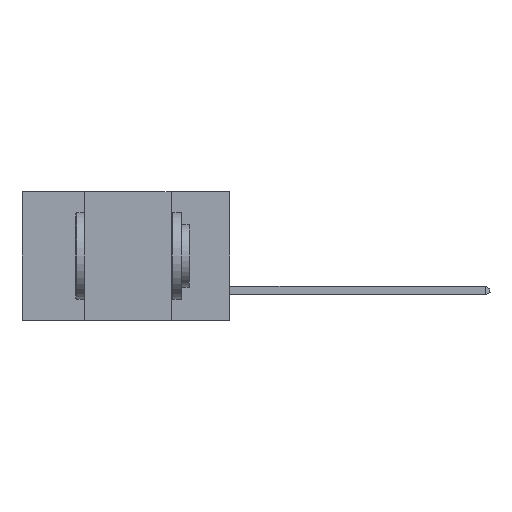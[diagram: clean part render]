
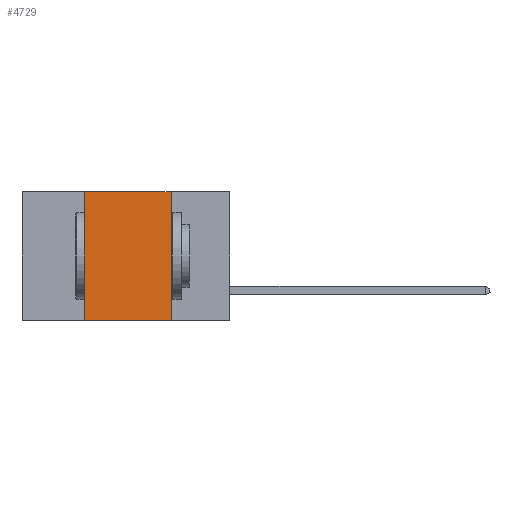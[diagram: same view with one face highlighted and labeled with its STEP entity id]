
A CAD part, left-side view. The second image highlights one B-rep face of the part: STEP entity #4729.
In plain terms, the highlighted planar face has unit normal (-1, 0, 0).
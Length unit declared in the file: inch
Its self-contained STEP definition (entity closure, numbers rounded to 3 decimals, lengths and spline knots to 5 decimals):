
#10 = ORIENTED_EDGE ( 'NONE', *, *, #11456, .F. ) ;
#204 = EDGE_CURVE ( 'NONE', #10013, #543, #9078, .T. ) ;
#543 = VERTEX_POINT ( 'NONE', #5342 ) ;
#908 = DIRECTION ( 'NONE',  ( 0., -1., 0. ) ) ;
#931 = DIRECTION ( 'NONE',  ( 0., 0., -1. ) ) ;
#1686 = DIRECTION ( 'NONE',  ( 0., 0., 1. ) ) ;
#1840 = CARTESIAN_POINT ( 'NONE',  ( 0., 0.42, -0.37 ) ) ;
#2018 = DIRECTION ( 'NONE',  ( 0., 0., -1. ) ) ;
#2090 = CARTESIAN_POINT ( 'NONE',  ( 0., 0.6, 0. ) ) ;
#2192 = VECTOR ( 'NONE', #7579, 39.37008 ) ;
#2396 = ORIENTED_EDGE ( 'NONE', *, *, #10674, .T. ) ;
#2533 = VECTOR ( 'NONE', #908, 39.37008 ) ;
#3276 = FACE_OUTER_BOUND ( 'NONE', #3877, .T. ) ;
#3305 = AXIS2_PLACEMENT_3D ( 'NONE', #2090, #7664, #2018 ) ;
#3877 = EDGE_LOOP ( 'NONE', ( #9782, #11064, #10, #2396 ) ) ;
#4577 = CARTESIAN_POINT ( 'NONE',  ( 0., 0.6, -0.37 ) ) ;
#4715 = CARTESIAN_POINT ( 'NONE',  ( 0., 0.6, 0. ) ) ;
#4729 = ADVANCED_FACE ( 'NONE', ( #3276 ), #10416, .F. ) ;
#4850 = LINE ( 'NONE', #4715, #2192 ) ;
#5342 = CARTESIAN_POINT ( 'NONE',  ( 0., 0.17, -0.37 ) ) ;
#5613 = CARTESIAN_POINT ( 'NONE',  ( 0., 0.17, 0. ) ) ;
#6871 = CARTESIAN_POINT ( 'NONE',  ( 0., 0.42, 0. ) ) ;
#7040 = EDGE_CURVE ( 'NONE', #7874, #10013, #4850, .T. ) ;
#7411 = LINE ( 'NONE', #4577, #2533 ) ;
#7579 = DIRECTION ( 'NONE',  ( 0., -1., 0. ) ) ;
#7664 = DIRECTION ( 'NONE',  ( 1., 0., 0. ) ) ;
#7874 = VERTEX_POINT ( 'NONE', #6871 ) ;
#8236 = CARTESIAN_POINT ( 'NONE',  ( 0., 0.17, 0. ) ) ;
#9078 = LINE ( 'NONE', #5613, #11303 ) ;
#9173 = CARTESIAN_POINT ( 'NONE',  ( 0., 0.42, 0. ) ) ;
#9782 = ORIENTED_EDGE ( 'NONE', *, *, #204, .F. ) ;
#9894 = VECTOR ( 'NONE', #1686, 39.37008 ) ;
#10013 = VERTEX_POINT ( 'NONE', #8236 ) ;
#10416 = PLANE ( 'NONE',  #3305 ) ;
#10486 = LINE ( 'NONE', #9173, #9894 ) ;
#10674 = EDGE_CURVE ( 'NONE', #11478, #543, #7411, .T. ) ;
#11064 = ORIENTED_EDGE ( 'NONE', *, *, #7040, .F. ) ;
#11303 = VECTOR ( 'NONE', #931, 39.37008 ) ;
#11456 = EDGE_CURVE ( 'NONE', #11478, #7874, #10486, .T. ) ;
#11478 = VERTEX_POINT ( 'NONE', #1840 ) ;
